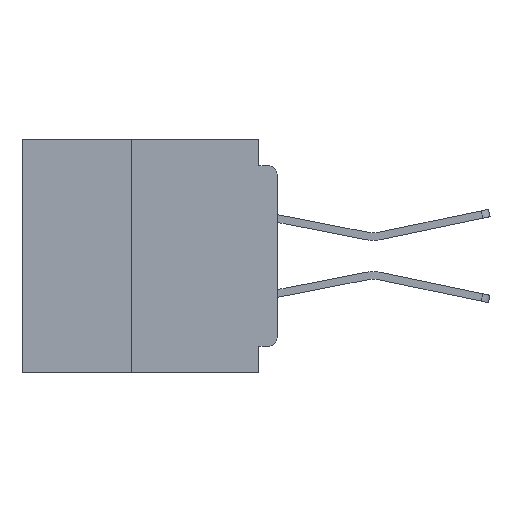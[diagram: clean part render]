
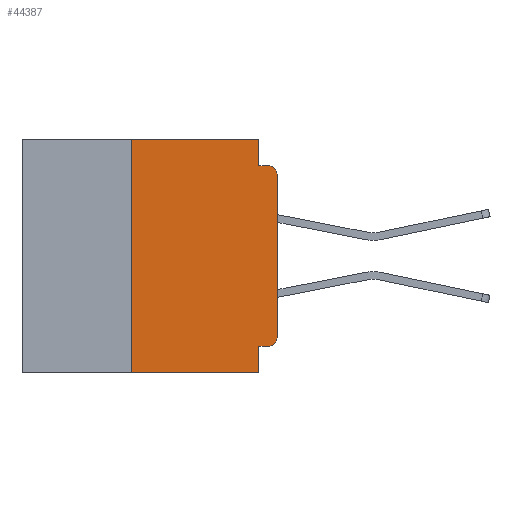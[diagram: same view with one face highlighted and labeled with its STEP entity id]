
A CAD part, left-side view. The second image highlights one B-rep face of the part: STEP entity #44387.
In plain terms, the highlighted planar face has unit normal (-1, 0, 0).
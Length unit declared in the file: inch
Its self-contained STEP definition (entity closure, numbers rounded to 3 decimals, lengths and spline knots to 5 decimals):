
#786 = CARTESIAN_POINT ( 'NONE',  ( 0., 0.437, 0. ) ) ;
#851 = VERTEX_POINT ( 'NONE', #38601 ) ;
#1565 = EDGE_CURVE ( 'NONE', #851, #5755, #22182, .T. ) ;
#2007 = VERTEX_POINT ( 'NONE', #55626 ) ;
#2262 = CARTESIAN_POINT ( 'NONE',  ( 0., 0.437, 0. ) ) ;
#3878 = CARTESIAN_POINT ( 'NONE',  ( 0., 0.031, -0.045 ) ) ;
#4784 = EDGE_CURVE ( 'NONE', #851, #41685, #44534, .T. ) ;
#4918 = CARTESIAN_POINT ( 'NONE',  ( 0., 0.25, 0. ) ) ;
#5345 = DIRECTION ( 'NONE',  ( 0., 0., -1. ) ) ;
#5525 = VERTEX_POINT ( 'NONE', #4918 ) ;
#5755 = VERTEX_POINT ( 'NONE', #20180 ) ;
#8158 = CARTESIAN_POINT ( 'NONE',  ( 0., 0.031, -0.4 ) ) ;
#8407 = DIRECTION ( 'NONE',  ( 0., 0., -1. ) ) ;
#8522 = LINE ( 'NONE', #8158, #19170 ) ;
#8906 = DIRECTION ( 'NONE',  ( -1., 0., 0. ) ) ;
#8970 = CARTESIAN_POINT ( 'NONE',  ( 0., 0.015, -0.34 ) ) ;
#9116 = VECTOR ( 'NONE', #43479, 39.37008 ) ;
#9425 = EDGE_CURVE ( 'NONE', #2007, #48802, #28688, .T. ) ;
#10511 = ORIENTED_EDGE ( 'NONE', *, *, #1565, .T. ) ;
#11702 = ORIENTED_EDGE ( 'NONE', *, *, #13513, .T. ) ;
#12150 = CARTESIAN_POINT ( 'NONE',  ( 0., 0., -0.06 ) ) ;
#13513 = EDGE_CURVE ( 'NONE', #5755, #43482, #42373, .T. ) ;
#14358 = CARTESIAN_POINT ( 'NONE',  ( 0., 0.031, 0. ) ) ;
#15565 = CARTESIAN_POINT ( 'NONE',  ( 0., 0.031, 0. ) ) ;
#15569 = EDGE_CURVE ( 'NONE', #24014, #30485, #18026, .T. ) ;
#15697 = DIRECTION ( 'NONE',  ( 0., 0., 1. ) ) ;
#17075 = CARTESIAN_POINT ( 'NONE',  ( 0., 0., -0.355 ) ) ;
#18026 = LINE ( 'NONE', #41931, #51712 ) ;
#18164 = FACE_OUTER_BOUND ( 'NONE', #31583, .T. ) ;
#18226 = AXIS2_PLACEMENT_3D ( 'NONE', #22924, #53533, #27381 ) ;
#19170 = VECTOR ( 'NONE', #34905, 39.37008 ) ;
#20180 = CARTESIAN_POINT ( 'NONE',  ( 0., 0., -0.34 ) ) ;
#20374 = EDGE_CURVE ( 'NONE', #43482, #30485, #26790, .T. ) ;
#22182 = CIRCLE ( 'NONE', #29788, 0.015 ) ;
#22785 = VECTOR ( 'NONE', #37809, 39.37008 ) ;
#22924 = CARTESIAN_POINT ( 'NONE',  ( 0., 0.015, -0.06 ) ) ;
#23189 = VECTOR ( 'NONE', #15697, 39.37008 ) ;
#24014 = VERTEX_POINT ( 'NONE', #3878 ) ;
#24185 = LINE ( 'NONE', #2262, #22785 ) ;
#26790 = CIRCLE ( 'NONE', #18226, 0.015 ) ;
#27319 = VECTOR ( 'NONE', #36716, 39.37008 ) ;
#27381 = DIRECTION ( 'NONE',  ( 0., 0., -1. ) ) ;
#27697 = ORIENTED_EDGE ( 'NONE', *, *, #20374, .T. ) ;
#27807 = PLANE ( 'NONE',  #56633 ) ;
#28415 = DIRECTION ( 'NONE',  ( 0., 0., 1. ) ) ;
#28688 = LINE ( 'NONE', #41102, #27319 ) ;
#29788 = AXIS2_PLACEMENT_3D ( 'NONE', #8970, #8906, #8407 ) ;
#30485 = VERTEX_POINT ( 'NONE', #36830 ) ;
#30795 = VECTOR ( 'NONE', #28415, 39.37008 ) ;
#31583 = EDGE_LOOP ( 'NONE', ( #11702, #27697, #43645, #54679, #36822, #38852, #54073, #42519, #41357, #10511 ) ) ;
#32216 = DIRECTION ( 'NONE',  ( 1., 0., 0. ) ) ;
#34853 = LINE ( 'NONE', #42125, #23189 ) ;
#34905 = DIRECTION ( 'NONE',  ( 0., 0., -1. ) ) ;
#36716 = DIRECTION ( 'NONE',  ( 0., -1., 0. ) ) ;
#36822 = ORIENTED_EDGE ( 'NONE', *, *, #48933, .F. ) ;
#36830 = CARTESIAN_POINT ( 'NONE',  ( 0., 0.015, -0.045 ) ) ;
#36989 = CARTESIAN_POINT ( 'NONE',  ( 0., 0., 0. ) ) ;
#37787 = DIRECTION ( 'NONE',  ( 0., 0., -1. ) ) ;
#37809 = DIRECTION ( 'NONE',  ( 0., -1., 0. ) ) ;
#38525 = LINE ( 'NONE', #15565, #48808 ) ;
#38601 = CARTESIAN_POINT ( 'NONE',  ( 0., 0.015, -0.355 ) ) ;
#38852 = ORIENTED_EDGE ( 'NONE', *, *, #51846, .F. ) ;
#39306 = VERTEX_POINT ( 'NONE', #14358 ) ;
#41102 = CARTESIAN_POINT ( 'NONE',  ( 0., 0.437, -0.4 ) ) ;
#41357 = ORIENTED_EDGE ( 'NONE', *, *, #4784, .F. ) ;
#41685 = VERTEX_POINT ( 'NONE', #48117 ) ;
#41931 = CARTESIAN_POINT ( 'NONE',  ( 0., 0., -0.045 ) ) ;
#42125 = CARTESIAN_POINT ( 'NONE',  ( 0., 0.25, -0.4 ) ) ;
#42373 = LINE ( 'NONE', #36989, #30795 ) ;
#42519 = ORIENTED_EDGE ( 'NONE', *, *, #49619, .F. ) ;
#43479 = DIRECTION ( 'NONE',  ( 0., 1., 0. ) ) ;
#43482 = VERTEX_POINT ( 'NONE', #12150 ) ;
#43645 = ORIENTED_EDGE ( 'NONE', *, *, #15569, .F. ) ;
#44387 = ADVANCED_FACE ( 'NONE', ( #18164 ), #27807, .F. ) ;
#44534 = LINE ( 'NONE', #17075, #9116 ) ;
#45881 = CARTESIAN_POINT ( 'NONE',  ( 0., 0.031, -0.4 ) ) ;
#46349 = DIRECTION ( 'NONE',  ( 0., -1., 0. ) ) ;
#47674 = EDGE_CURVE ( 'NONE', #39306, #24014, #38525, .T. ) ;
#48117 = CARTESIAN_POINT ( 'NONE',  ( 0., 0.031, -0.355 ) ) ;
#48802 = VERTEX_POINT ( 'NONE', #45881 ) ;
#48808 = VECTOR ( 'NONE', #37787, 39.37008 ) ;
#48933 = EDGE_CURVE ( 'NONE', #5525, #39306, #24185, .T. ) ;
#49619 = EDGE_CURVE ( 'NONE', #41685, #48802, #8522, .T. ) ;
#51712 = VECTOR ( 'NONE', #46349, 39.37008 ) ;
#51846 = EDGE_CURVE ( 'NONE', #2007, #5525, #34853, .T. ) ;
#53533 = DIRECTION ( 'NONE',  ( -1., 0., 0. ) ) ;
#54073 = ORIENTED_EDGE ( 'NONE', *, *, #9425, .T. ) ;
#54679 = ORIENTED_EDGE ( 'NONE', *, *, #47674, .F. ) ;
#55626 = CARTESIAN_POINT ( 'NONE',  ( 0., 0.25, -0.4 ) ) ;
#56633 = AXIS2_PLACEMENT_3D ( 'NONE', #786, #32216, #5345 ) ;
